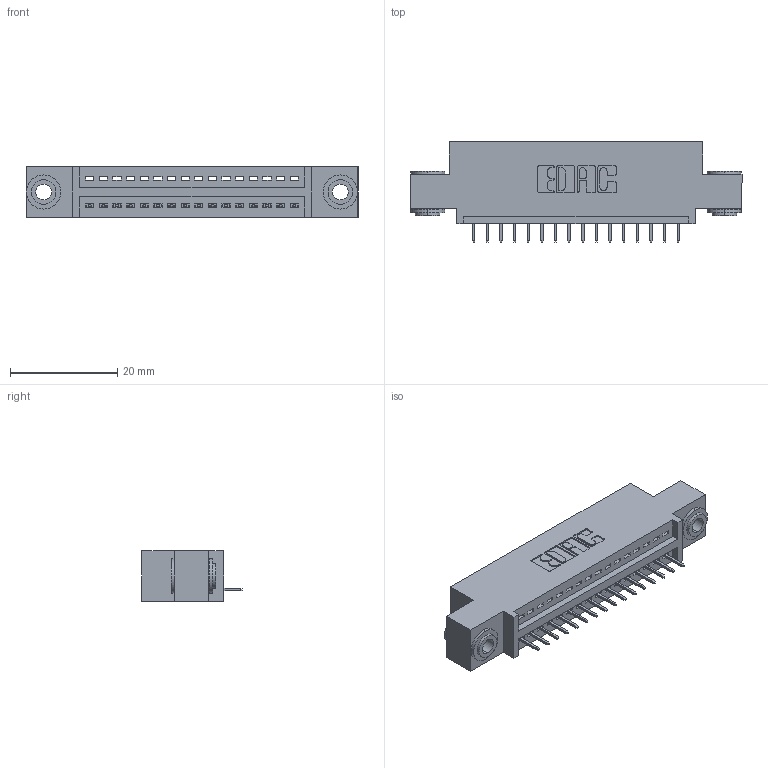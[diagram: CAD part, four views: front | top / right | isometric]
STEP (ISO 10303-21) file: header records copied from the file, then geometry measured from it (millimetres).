
FILE_DESCRIPTION (( 'STEP AP203' ), '1' );
FILE_NAME ('895-016-525-403.STEP', '2020-09-25T04:58:14', ( '' ), ( '' ), 'SwSTEP 2.0', 'SolidWorks 2020', '' );
FILE_SCHEMA (( 'CONFIG_CONTROL_DESIGN' ));
Length unit declared in the file: inch
Products named in the file (4): 345-292-001_345-293-125; 345-250-002_345-250-002-102; 895-016-525-403; 845 Part_0.110 Offset - 0.156 Dia-TH
Assembly tree (19 placements, depth 2):
  895-016-525-403
    845 Part_0.110 Offset - 0.156 Dia-TH
    345-292-001_345-293-125  x16
    345-250-002_345-250-002-102  x2
Bounding box: 61.85 x 18.72 x 9.4 mm (x, y, z)
Volume: 5542.2 mm3; surface area: 7090.2 mm2
Topology: 19 solids, 19 shells, 1160 faces, 3309 edges, 2138 vertices
Faces by surface type: plane 830, cylinder 322, cone 8
Entity records: 16398 total; most frequent: CARTESIAN_POINT 2819, ORIENTED_EDGE 2762, DIRECTION 2531, EDGE_CURVE 1381, VECTOR 1165, LINE 1165, VERTEX_POINT 914, AXIS2_PLACEMENT_3D 683
